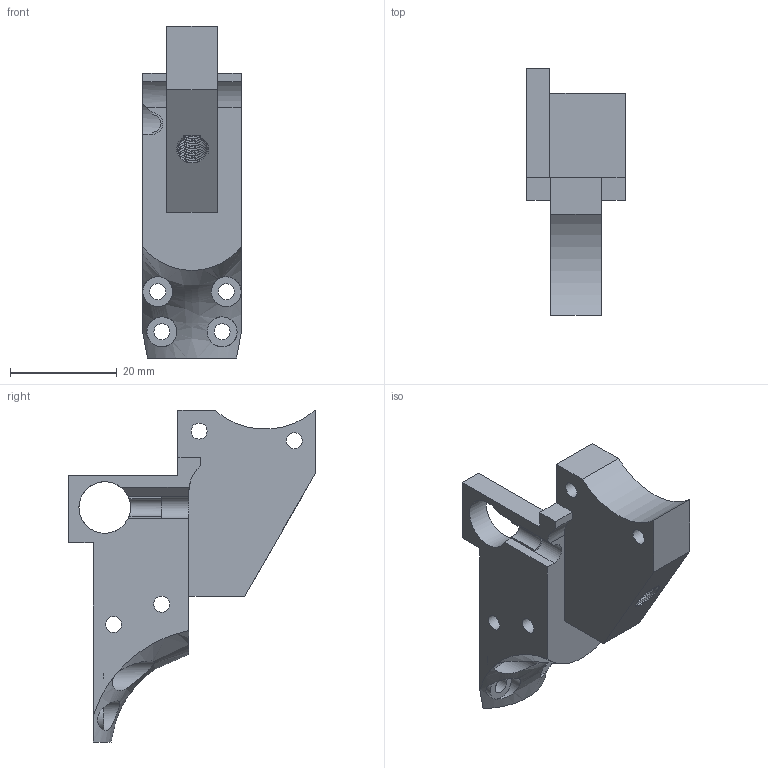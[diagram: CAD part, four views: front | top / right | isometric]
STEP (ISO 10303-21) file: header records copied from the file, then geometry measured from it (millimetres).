
FILE_DESCRIPTION(/* description */ (''),/* implementation_level */ '2;1');
FILE_NAME(/* name */ 'FCU Rear Joiner Type 2.step',/* time_stamp */ '2024-01-16T15:55:28-05:00',/* author */ (''),/* organization */ (''),/* preprocessor_version */ 'ST-DEVELOPER v20',/* originating_system */ 'Autodesk Translation Framework v12.14.0.127',/* authorisation */ '');
FILE_SCHEMA (('AUTOMOTIVE_DESIGN { 1 0 10303 214 3 1 1 }'));
Length unit declared in the file: inch
Products named in the file (1): FCU Rear Joiner Type 2
Bounding box: 18.44 x 46.1 x 62.07 mm (x, y, z)
Volume: 12885.5 mm3; surface area: 7030.1 mm2
Topology: 1 solids, 1 shells, 177 faces, 514 edges, 342 vertices
Faces by surface type: cylinder 81, bspline 62, plane 34
Full cylindrical faces by diameter (mm): 3 x8, 5.6 x2, 9.652 x1
Entity records: 9432 total; most frequent: CARTESIAN_POINT 5321, ORIENTED_EDGE 1028, DIRECTION 544, EDGE_CURVE 514, VERTEX_POINT 342, B_SPLINE_CURVE_WITH_KNOTS 260, EDGE_LOOP 200, LINE 196
